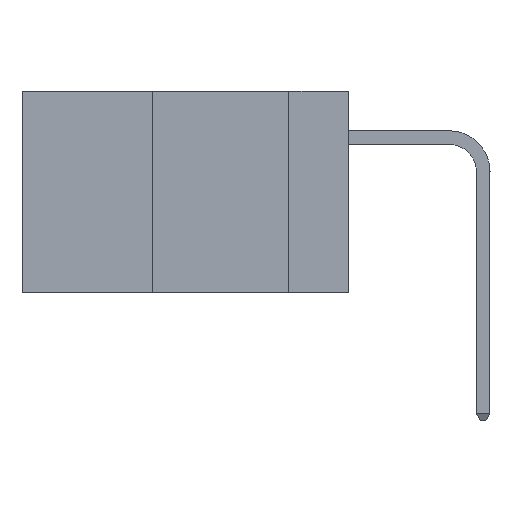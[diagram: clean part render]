
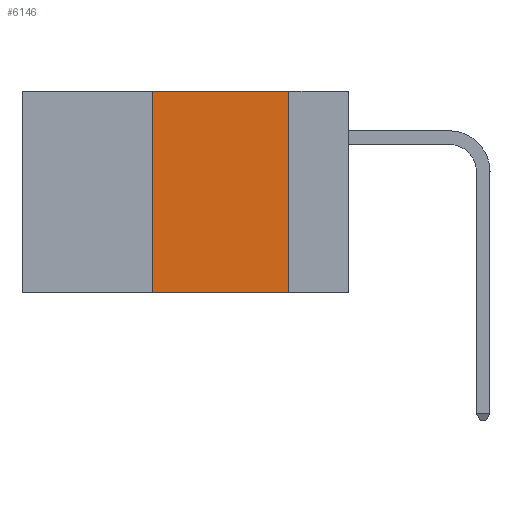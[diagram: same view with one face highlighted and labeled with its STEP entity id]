
A CAD part, left-side view. The second image highlights one B-rep face of the part: STEP entity #6146.
In plain terms, the highlighted planar face has unit normal (-1, 0, 0).
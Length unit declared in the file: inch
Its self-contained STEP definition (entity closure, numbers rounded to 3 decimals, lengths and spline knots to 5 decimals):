
#111 = VERTEX_POINT ( 'NONE', #16242 ) ;
#1948 = EDGE_LOOP ( 'NONE', ( #29543, #20363, #17280, #6743 ) ) ;
#3585 = VERTEX_POINT ( 'NONE', #16707 ) ;
#4564 = PLANE ( 'NONE',  #31858 ) ;
#4736 = FACE_OUTER_BOUND ( 'NONE', #1948, .T. ) ;
#6146 = ADVANCED_FACE ( 'NONE', ( #4736 ), #4564, .F. ) ;
#6743 = ORIENTED_EDGE ( 'NONE', *, *, #15611, .T. ) ;
#7655 = EDGE_CURVE ( 'NONE', #35277, #35769, #29671, .T. ) ;
#8642 = VECTOR ( 'NONE', #32795, 39.37008 ) ;
#10169 = VECTOR ( 'NONE', #29040, 39.37008 ) ;
#11923 = EDGE_CURVE ( 'NONE', #35769, #3585, #25041, .T. ) ;
#12299 = DIRECTION ( 'NONE',  ( 0., 0., 1. ) ) ;
#12342 = VECTOR ( 'NONE', #12299, 39.37008 ) ;
#12550 = CARTESIAN_POINT ( 'NONE',  ( 0., 0.36, -0.37 ) ) ;
#13711 = CARTESIAN_POINT ( 'NONE',  ( 0., 0.6, -0.37 ) ) ;
#13873 = DIRECTION ( 'NONE',  ( 1., 0., 0. ) ) ;
#15611 = EDGE_CURVE ( 'NONE', #35277, #111, #18414, .T. ) ;
#16242 = CARTESIAN_POINT ( 'NONE',  ( 0., 0.11, -0.37 ) ) ;
#16707 = CARTESIAN_POINT ( 'NONE',  ( 0., 0.11, 0. ) ) ;
#17280 = ORIENTED_EDGE ( 'NONE', *, *, #7655, .F. ) ;
#18414 = LINE ( 'NONE', #13711, #10169 ) ;
#20363 = ORIENTED_EDGE ( 'NONE', *, *, #11923, .F. ) ;
#23042 = CARTESIAN_POINT ( 'NONE',  ( 0., 0.6, 0. ) ) ;
#24546 = CARTESIAN_POINT ( 'NONE',  ( 0., 0.11, 0. ) ) ;
#25041 = LINE ( 'NONE', #29729, #8642 ) ;
#25198 = VECTOR ( 'NONE', #36812, 39.37008 ) ;
#26577 = EDGE_CURVE ( 'NONE', #3585, #111, #33359, .T. ) ;
#29040 = DIRECTION ( 'NONE',  ( 0., -1., 0. ) ) ;
#29543 = ORIENTED_EDGE ( 'NONE', *, *, #26577, .F. ) ;
#29671 = LINE ( 'NONE', #30705, #12342 ) ;
#29729 = CARTESIAN_POINT ( 'NONE',  ( 0., 0.6, 0. ) ) ;
#30705 = CARTESIAN_POINT ( 'NONE',  ( 0., 0.36, 0. ) ) ;
#31858 = AXIS2_PLACEMENT_3D ( 'NONE', #23042, #13873, #35339 ) ;
#32795 = DIRECTION ( 'NONE',  ( 0., -1., 0. ) ) ;
#33359 = LINE ( 'NONE', #24546, #25198 ) ;
#35277 = VERTEX_POINT ( 'NONE', #12550 ) ;
#35339 = DIRECTION ( 'NONE',  ( 0., 0., -1. ) ) ;
#35769 = VERTEX_POINT ( 'NONE', #36378 ) ;
#36378 = CARTESIAN_POINT ( 'NONE',  ( 0., 0.36, 0. ) ) ;
#36812 = DIRECTION ( 'NONE',  ( 0., 0., -1. ) ) ;
